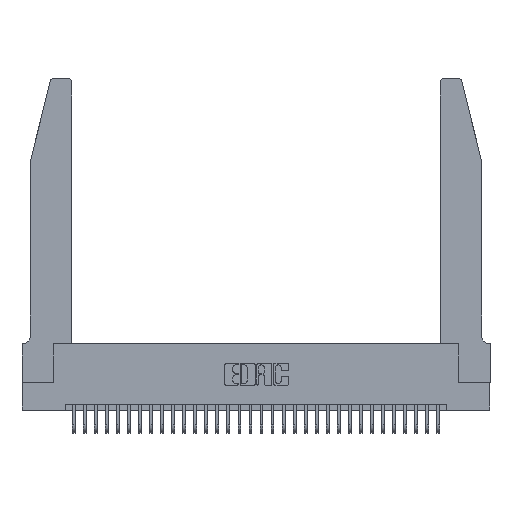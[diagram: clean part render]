
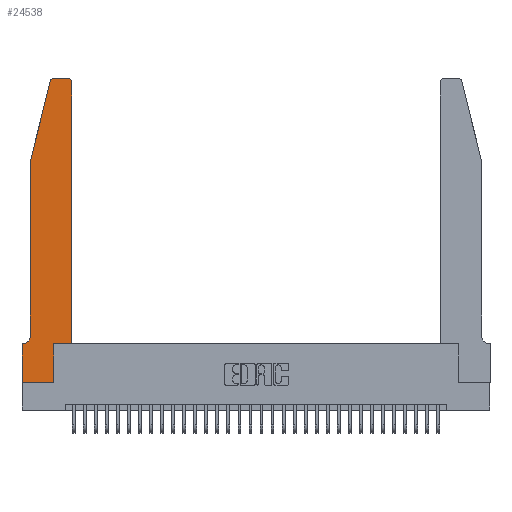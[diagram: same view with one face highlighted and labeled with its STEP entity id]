
A CAD part, top view. The second image highlights one B-rep face of the part: STEP entity #24538.
In plain terms, the highlighted planar face has unit normal (0, 0, 1).
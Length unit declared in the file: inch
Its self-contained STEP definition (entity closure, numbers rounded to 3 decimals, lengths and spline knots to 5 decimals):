
#231 = DIRECTION ( 'NONE',  ( 0., 0., -1. ) ) ;
#240 = CARTESIAN_POINT ( 'NONE',  ( 0.4505, 0.35, 0.37 ) ) ;
#1582 = DIRECTION ( 'NONE',  ( 0., 0., 1. ) ) ;
#1897 = VERTEX_POINT ( 'NONE', #19794 ) ;
#2278 = VERTEX_POINT ( 'NONE', #8165 ) ;
#2411 = VECTOR ( 'NONE', #20250, 39.37008 ) ;
#2532 = VECTOR ( 'NONE', #31396, 39.37008 ) ;
#2623 = LINE ( 'NONE', #11042, #17505 ) ;
#4675 = ORIENTED_EDGE ( 'NONE', *, *, #11302, .T. ) ;
#4732 = ORIENTED_EDGE ( 'NONE', *, *, #13763, .T. ) ;
#4781 = LINE ( 'NONE', #19641, #18031 ) ;
#5088 = VERTEX_POINT ( 'NONE', #31376 ) ;
#5151 = CARTESIAN_POINT ( 'NONE',  ( 0.284, 2.75, 0.37 ) ) ;
#5339 = DIRECTION ( 'NONE',  ( 1., 0., 0. ) ) ;
#5695 = LINE ( 'NONE', #26596, #25980 ) ;
#6026 = PLANE ( 'NONE',  #28830 ) ;
#6229 = CIRCLE ( 'NONE', #25224, 0.03 ) ;
#6405 = DIRECTION ( 'NONE',  ( 0., -1., 0. ) ) ;
#7316 = VERTEX_POINT ( 'NONE', #29851 ) ;
#7791 = EDGE_CURVE ( 'NONE', #21240, #32765, #19857, .T. ) ;
#8165 = CARTESIAN_POINT ( 'NONE',  ( 0.25487, 2.72718, 0.37 ) ) ;
#8675 = CARTESIAN_POINT ( 'NONE',  ( 0., 0.35, 0.37 ) ) ;
#8693 = LINE ( 'NONE', #12984, #2532 ) ;
#8719 = EDGE_CURVE ( 'NONE', #30638, #21240, #20626, .T. ) ;
#9933 = VERTEX_POINT ( 'NONE', #28523 ) ;
#10925 = ORIENTED_EDGE ( 'NONE', *, *, #25254, .T. ) ;
#11042 = CARTESIAN_POINT ( 'NONE',  ( 0., 0., 0.37 ) ) ;
#11302 = EDGE_CURVE ( 'NONE', #5088, #23568, #5695, .T. ) ;
#11370 = DIRECTION ( 'NONE',  ( 1., 0., 0. ) ) ;
#11384 = ORIENTED_EDGE ( 'NONE', *, *, #22036, .T. ) ;
#11667 = DIRECTION ( 'NONE',  ( 0., 0., 1. ) ) ;
#12720 = CARTESIAN_POINT ( 'NONE',  ( 0., 0.35, 0.37 ) ) ;
#12788 = VECTOR ( 'NONE', #22964, 39.37008 ) ;
#12791 = EDGE_CURVE ( 'NONE', #7316, #1897, #4781, .T. ) ;
#12984 = CARTESIAN_POINT ( 'NONE',  ( 0.4505, 0.35, 0.37 ) ) ;
#13763 = EDGE_CURVE ( 'NONE', #1897, #19467, #18377, .T. ) ;
#14982 = EDGE_CURVE ( 'NONE', #21542, #9933, #2623, .T. ) ;
#15964 = EDGE_CURVE ( 'NONE', #23568, #2278, #6229, .T. ) ;
#16073 = CARTESIAN_POINT ( 'NONE',  ( 0.0055, 0.42, 0.37 ) ) ;
#16078 = DIRECTION ( 'NONE',  ( -1., 0., 0. ) ) ;
#17403 = CARTESIAN_POINT ( 'NONE',  ( 0.284, 2.72, 0.37 ) ) ;
#17505 = VECTOR ( 'NONE', #19017, 39.37008 ) ;
#17568 = CARTESIAN_POINT ( 'NONE',  ( 0.0755, 2., 0.37 ) ) ;
#17653 = CARTESIAN_POINT ( 'NONE',  ( 0.2865, 0.35, 0.37 ) ) ;
#18031 = VECTOR ( 'NONE', #6405, 39.37008 ) ;
#18377 = CIRCLE ( 'NONE', #18571, 0.07 ) ;
#18540 = CARTESIAN_POINT ( 'NONE',  ( 0.4505, 0.35, 0.37 ) ) ;
#18544 = VECTOR ( 'NONE', #30509, 39.37008 ) ;
#18571 = AXIS2_PLACEMENT_3D ( 'NONE', #16073, #231, #18739 ) ;
#18739 = DIRECTION ( 'NONE',  ( -1., 0., 0. ) ) ;
#18847 = ORIENTED_EDGE ( 'NONE', *, *, #31941, .T. ) ;
#19017 = DIRECTION ( 'NONE',  ( 0., -1., 0. ) ) ;
#19195 = ORIENTED_EDGE ( 'NONE', *, *, #15964, .T. ) ;
#19467 = VERTEX_POINT ( 'NONE', #26131 ) ;
#19531 = CARTESIAN_POINT ( 'NONE',  ( 0.2865, 0.35, 0.37 ) ) ;
#19641 = CARTESIAN_POINT ( 'NONE',  ( 0.0755, 2., 0.37 ) ) ;
#19741 = EDGE_CURVE ( 'NONE', #31884, #5088, #24892, .T. ) ;
#19794 = CARTESIAN_POINT ( 'NONE',  ( 0.0755, 0.42, 0.37 ) ) ;
#19857 = LINE ( 'NONE', #18540, #26036 ) ;
#20078 = DIRECTION ( 'NONE',  ( 1., 0., 0. ) ) ;
#20130 = ORIENTED_EDGE ( 'NONE', *, *, #7791, .T. ) ;
#20211 = VECTOR ( 'NONE', #20797, 39.37008 ) ;
#20250 = DIRECTION ( 'NONE',  ( -0.239, -0.971, 0. ) ) ;
#20266 = AXIS2_PLACEMENT_3D ( 'NONE', #27462, #11667, #30106 ) ;
#20522 = ORIENTED_EDGE ( 'NONE', *, *, #8719, .T. ) ;
#20626 = LINE ( 'NONE', #17653, #12788 ) ;
#20797 = DIRECTION ( 'NONE',  ( 1., 0., 0. ) ) ;
#20866 = CARTESIAN_POINT ( 'NONE',  ( 0.2865, 0., 0.37 ) ) ;
#21006 = ORIENTED_EDGE ( 'NONE', *, *, #19741, .T. ) ;
#21059 = LINE ( 'NONE', #28713, #20211 ) ;
#21240 = VERTEX_POINT ( 'NONE', #19531 ) ;
#21542 = VERTEX_POINT ( 'NONE', #12720 ) ;
#22036 = EDGE_CURVE ( 'NONE', #19467, #21542, #33377, .T. ) ;
#22916 = EDGE_CURVE ( 'NONE', #32765, #31884, #8693, .T. ) ;
#22964 = DIRECTION ( 'NONE',  ( 0., 1., 0. ) ) ;
#23495 = LINE ( 'NONE', #17568, #2411 ) ;
#23568 = VERTEX_POINT ( 'NONE', #5151 ) ;
#23945 = FACE_OUTER_BOUND ( 'NONE', #29652, .T. ) ;
#24538 = ADVANCED_FACE ( 'NONE', ( #23945 ), #6026, .T. ) ;
#24892 = CIRCLE ( 'NONE', #20266, 0.03 ) ;
#25224 = AXIS2_PLACEMENT_3D ( 'NONE', #17403, #1582, #20078 ) ;
#25254 = EDGE_CURVE ( 'NONE', #2278, #7316, #23495, .T. ) ;
#25980 = VECTOR ( 'NONE', #16078, 39.37008 ) ;
#26036 = VECTOR ( 'NONE', #5339, 39.37008 ) ;
#26131 = CARTESIAN_POINT ( 'NONE',  ( 0.0055, 0.35, 0.37 ) ) ;
#26596 = CARTESIAN_POINT ( 'NONE',  ( 0.2605, 2.75, 0.37 ) ) ;
#26726 = ORIENTED_EDGE ( 'NONE', *, *, #22916, .T. ) ;
#27082 = ORIENTED_EDGE ( 'NONE', *, *, #14982, .T. ) ;
#27174 = DIRECTION ( 'NONE',  ( 0., 0., 1. ) ) ;
#27462 = CARTESIAN_POINT ( 'NONE',  ( 0.4205, 2.72, 0.37 ) ) ;
#27864 = CARTESIAN_POINT ( 'NONE',  ( 0.0755, 0.35, 0.37 ) ) ;
#28488 = CARTESIAN_POINT ( 'NONE',  ( 0.4505, 2.72, 0.37 ) ) ;
#28523 = CARTESIAN_POINT ( 'NONE',  ( 0., 0., 0.37 ) ) ;
#28713 = CARTESIAN_POINT ( 'NONE',  ( 0., 0., 0.37 ) ) ;
#28830 = AXIS2_PLACEMENT_3D ( 'NONE', #8675, #27174, #11370 ) ;
#29652 = EDGE_LOOP ( 'NONE', ( #4675, #19195, #10925, #31586, #4732, #11384, #27082, #18847, #20522, #20130, #26726, #21006 ) ) ;
#29851 = CARTESIAN_POINT ( 'NONE',  ( 0.0755, 2., 0.37 ) ) ;
#30106 = DIRECTION ( 'NONE',  ( 1., 0., 0. ) ) ;
#30509 = DIRECTION ( 'NONE',  ( -1., 0., 0. ) ) ;
#30638 = VERTEX_POINT ( 'NONE', #20866 ) ;
#31376 = CARTESIAN_POINT ( 'NONE',  ( 0.4205, 2.75, 0.37 ) ) ;
#31396 = DIRECTION ( 'NONE',  ( 0., 1., 0. ) ) ;
#31586 = ORIENTED_EDGE ( 'NONE', *, *, #12791, .T. ) ;
#31884 = VERTEX_POINT ( 'NONE', #28488 ) ;
#31941 = EDGE_CURVE ( 'NONE', #9933, #30638, #21059, .T. ) ;
#32765 = VERTEX_POINT ( 'NONE', #240 ) ;
#33377 = LINE ( 'NONE', #27864, #18544 ) ;
